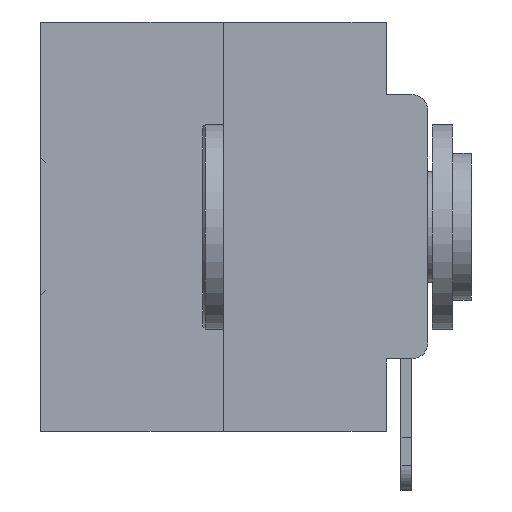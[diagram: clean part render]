
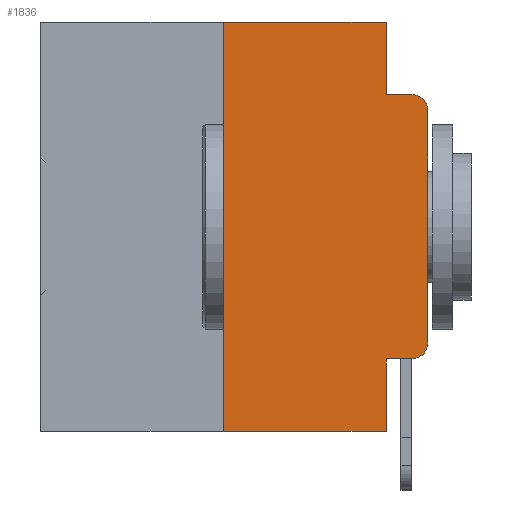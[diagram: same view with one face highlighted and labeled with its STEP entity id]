
A CAD part, left-side view. The second image highlights one B-rep face of the part: STEP entity #1836.
In plain terms, the highlighted planar face has unit normal (-1, 0, 0).
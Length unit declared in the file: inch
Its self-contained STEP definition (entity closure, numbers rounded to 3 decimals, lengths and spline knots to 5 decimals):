
#199 = CARTESIAN_POINT ( 'NONE',  ( 0., 0., -0.3915 ) ) ;
#976 = DIRECTION ( 'NONE',  ( -1., 0., 0. ) ) ;
#1116 = EDGE_CURVE ( 'NONE', #24588, #33378, #16121, .T. ) ;
#1428 = CARTESIAN_POINT ( 'NONE',  ( 0., 0.051, 0. ) ) ;
#1795 = ORIENTED_EDGE ( 'NONE', *, *, #9932, .T. ) ;
#1836 = ADVANCED_FACE ( 'NONE', ( #4830 ), #18016, .F. ) ;
#2303 = ORIENTED_EDGE ( 'NONE', *, *, #28081, .F. ) ;
#2912 = ORIENTED_EDGE ( 'NONE', *, *, #26934, .F. ) ;
#3360 = VERTEX_POINT ( 'NONE', #6543 ) ;
#3391 = VERTEX_POINT ( 'NONE', #27644 ) ;
#3738 = LINE ( 'NONE', #1428, #17531 ) ;
#4338 = DIRECTION ( 'NONE',  ( 1., 0., 0. ) ) ;
#4399 = LINE ( 'NONE', #5009, #18920 ) ;
#4416 = DIRECTION ( 'NONE',  ( 0., 0., -1. ) ) ;
#4501 = AXIS2_PLACEMENT_3D ( 'NONE', #15057, #32582, #17656 ) ;
#4830 = FACE_OUTER_BOUND ( 'NONE', #24537, .T. ) ;
#5009 = CARTESIAN_POINT ( 'NONE',  ( 0., 0.051, -0.0885 ) ) ;
#5700 = CARTESIAN_POINT ( 'NONE',  ( 0., 0.051, 0. ) ) ;
#6319 = VECTOR ( 'NONE', #14519, 39.37008 ) ;
#6321 = VECTOR ( 'NONE', #6688, 39.37008 ) ;
#6543 = CARTESIAN_POINT ( 'NONE',  ( 0., 0.02, -0.4115 ) ) ;
#6688 = DIRECTION ( 'NONE',  ( 0., -1., 0. ) ) ;
#6845 = VERTEX_POINT ( 'NONE', #23069 ) ;
#6998 = EDGE_CURVE ( 'NONE', #33378, #3391, #4399, .T. ) ;
#7854 = VECTOR ( 'NONE', #30071, 39.37008 ) ;
#8921 = EDGE_CURVE ( 'NONE', #14808, #3391, #10065, .T. ) ;
#9469 = CARTESIAN_POINT ( 'NONE',  ( 0., 0.473, -0.5 ) ) ;
#9739 = LINE ( 'NONE', #29691, #23617 ) ;
#9932 = EDGE_CURVE ( 'NONE', #28958, #14126, #21455, .T. ) ;
#10006 = CARTESIAN_POINT ( 'NONE',  ( 0., 0.473, 0. ) ) ;
#10065 = CIRCLE ( 'NONE', #31827, 0.02 ) ;
#10787 = ORIENTED_EDGE ( 'NONE', *, *, #8921, .T. ) ;
#11466 = ORIENTED_EDGE ( 'NONE', *, *, #28653, .F. ) ;
#11647 = ORIENTED_EDGE ( 'NONE', *, *, #6998, .F. ) ;
#14126 = VERTEX_POINT ( 'NONE', #21048 ) ;
#14519 = DIRECTION ( 'NONE',  ( 0., 0., 1. ) ) ;
#14808 = VERTEX_POINT ( 'NONE', #22895 ) ;
#15057 = CARTESIAN_POINT ( 'NONE',  ( 0., 0.02, -0.3915 ) ) ;
#15168 = LINE ( 'NONE', #20025, #7854 ) ;
#16121 = LINE ( 'NONE', #5700, #28752 ) ;
#16190 = EDGE_CURVE ( 'NONE', #22720, #14808, #15168, .T. ) ;
#16653 = DIRECTION ( 'NONE',  ( 0., 0., -1. ) ) ;
#17174 = DIRECTION ( 'NONE',  ( 0., -1., 0. ) ) ;
#17253 = CARTESIAN_POINT ( 'NONE',  ( 0., 0.25, 0. ) ) ;
#17464 = VECTOR ( 'NONE', #29199, 39.37008 ) ;
#17531 = VECTOR ( 'NONE', #4416, 39.37008 ) ;
#17597 = AXIS2_PLACEMENT_3D ( 'NONE', #10006, #4338, #23101 ) ;
#17656 = DIRECTION ( 'NONE',  ( 0., 0., -1. ) ) ;
#17692 = CARTESIAN_POINT ( 'NONE',  ( 0., 0.02, -0.1085 ) ) ;
#18016 = PLANE ( 'NONE',  #17597 ) ;
#18278 = CARTESIAN_POINT ( 'NONE',  ( 0., 0.25, -0.5 ) ) ;
#18570 = EDGE_CURVE ( 'NONE', #3360, #22720, #29379, .T. ) ;
#18671 = ORIENTED_EDGE ( 'NONE', *, *, #23652, .T. ) ;
#18920 = VECTOR ( 'NONE', #31079, 39.37008 ) ;
#18991 = ORIENTED_EDGE ( 'NONE', *, *, #18570, .T. ) ;
#20025 = CARTESIAN_POINT ( 'NONE',  ( 0., 0., 0. ) ) ;
#20248 = DIRECTION ( 'NONE',  ( 0., 0., -1. ) ) ;
#20488 = CARTESIAN_POINT ( 'NONE',  ( 0., 0.051, -0.0885 ) ) ;
#21048 = CARTESIAN_POINT ( 'NONE',  ( 0., 0.051, -0.5 ) ) ;
#21455 = LINE ( 'NONE', #9469, #6321 ) ;
#21676 = CARTESIAN_POINT ( 'NONE',  ( 0., 0.051, -0.4115 ) ) ;
#22720 = VERTEX_POINT ( 'NONE', #199 ) ;
#22895 = CARTESIAN_POINT ( 'NONE',  ( 0., 0., -0.1085 ) ) ;
#23069 = CARTESIAN_POINT ( 'NONE',  ( 0., 0.25, 0. ) ) ;
#23101 = DIRECTION ( 'NONE',  ( 0., 0., -1. ) ) ;
#23437 = VERTEX_POINT ( 'NONE', #21676 ) ;
#23617 = VECTOR ( 'NONE', #17174, 39.37008 ) ;
#23652 = EDGE_CURVE ( 'NONE', #23437, #3360, #9739, .T. ) ;
#24537 = EDGE_LOOP ( 'NONE', ( #24757, #10787, #11647, #25397, #2303, #11466, #1795, #2912, #18671, #18991 ) ) ;
#24588 = VERTEX_POINT ( 'NONE', #30096 ) ;
#24757 = ORIENTED_EDGE ( 'NONE', *, *, #16190, .T. ) ;
#25397 = ORIENTED_EDGE ( 'NONE', *, *, #1116, .F. ) ;
#25724 = LINE ( 'NONE', #17253, #6319 ) ;
#26670 = CARTESIAN_POINT ( 'NONE',  ( 0., 0.473, 0. ) ) ;
#26934 = EDGE_CURVE ( 'NONE', #23437, #14126, #3738, .T. ) ;
#27644 = CARTESIAN_POINT ( 'NONE',  ( 0., 0.02, -0.0885 ) ) ;
#28081 = EDGE_CURVE ( 'NONE', #6845, #24588, #30812, .T. ) ;
#28653 = EDGE_CURVE ( 'NONE', #28958, #6845, #25724, .T. ) ;
#28752 = VECTOR ( 'NONE', #16653, 39.37008 ) ;
#28958 = VERTEX_POINT ( 'NONE', #18278 ) ;
#29199 = DIRECTION ( 'NONE',  ( 0., -1., 0. ) ) ;
#29379 = CIRCLE ( 'NONE', #4501, 0.02 ) ;
#29691 = CARTESIAN_POINT ( 'NONE',  ( 0., 0.051, -0.4115 ) ) ;
#30071 = DIRECTION ( 'NONE',  ( 0., 0., 1. ) ) ;
#30096 = CARTESIAN_POINT ( 'NONE',  ( 0., 0.051, 0. ) ) ;
#30812 = LINE ( 'NONE', #26670, #17464 ) ;
#31079 = DIRECTION ( 'NONE',  ( 0., -1., 0. ) ) ;
#31827 = AXIS2_PLACEMENT_3D ( 'NONE', #17692, #976, #20248 ) ;
#32582 = DIRECTION ( 'NONE',  ( -1., 0., 0. ) ) ;
#33378 = VERTEX_POINT ( 'NONE', #20488 ) ;
